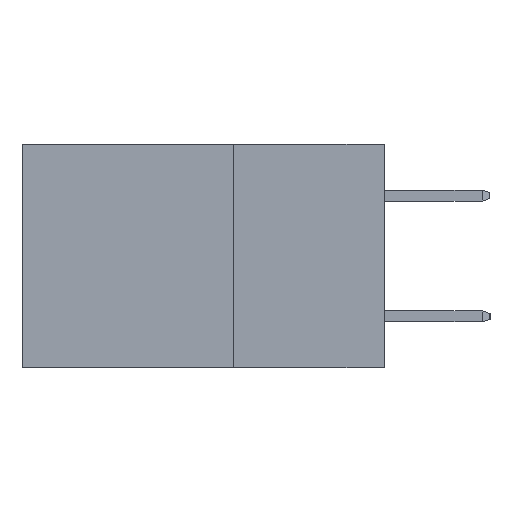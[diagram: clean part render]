
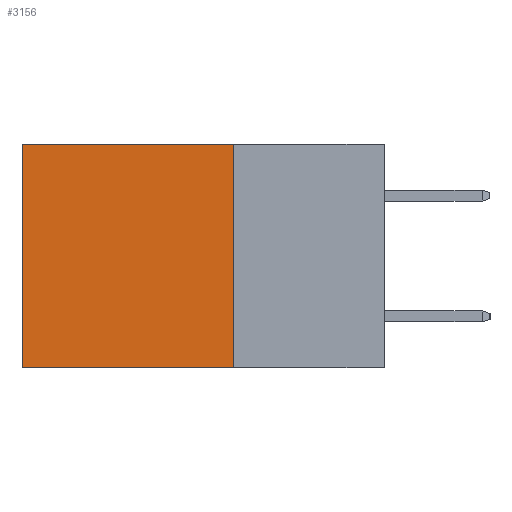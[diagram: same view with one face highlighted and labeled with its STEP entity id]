
A CAD part, left-side view. The second image highlights one B-rep face of the part: STEP entity #3156.
In plain terms, the highlighted planar face has unit normal (-1, 0, 0).
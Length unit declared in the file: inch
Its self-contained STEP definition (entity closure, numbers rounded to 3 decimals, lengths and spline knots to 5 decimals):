
#375 = ORIENTED_EDGE ( 'NONE', *, *, #1338, .T. ) ;
#456 = FACE_OUTER_BOUND ( 'NONE', #4893, .T. ) ;
#567 = DIRECTION ( 'NONE',  ( 0., 0., -1. ) ) ;
#1302 = DIRECTION ( 'NONE',  ( 1., 0., 0. ) ) ;
#1338 = EDGE_CURVE ( 'NONE', #3734, #2623, #2276, .T. ) ;
#1370 = CARTESIAN_POINT ( 'NONE',  ( 0.2615, 0.25, -0.37 ) ) ;
#1402 = VERTEX_POINT ( 'NONE', #6561 ) ;
#1409 = CARTESIAN_POINT ( 'NONE',  ( 0.2615, 0.25, 0. ) ) ;
#1435 = LINE ( 'NONE', #5054, #8711 ) ;
#1612 = EDGE_CURVE ( 'NONE', #2623, #4270, #5603, .T. ) ;
#1864 = DIRECTION ( 'NONE',  ( 0., 1., 0. ) ) ;
#2276 = LINE ( 'NONE', #5927, #5505 ) ;
#2623 = VERTEX_POINT ( 'NONE', #6834 ) ;
#3156 = ADVANCED_FACE ( 'NONE', ( #456 ), #7537, .F. ) ;
#3718 = VECTOR ( 'NONE', #5044, 39.37008 ) ;
#3734 = VERTEX_POINT ( 'NONE', #1409 ) ;
#4270 = VERTEX_POINT ( 'NONE', #4678 ) ;
#4388 = ORIENTED_EDGE ( 'NONE', *, *, #7783, .F. ) ;
#4629 = EDGE_CURVE ( 'NONE', #1402, #4270, #5745, .T. ) ;
#4678 = CARTESIAN_POINT ( 'NONE',  ( 0.2615, 0.6, -0.37 ) ) ;
#4829 = CARTESIAN_POINT ( 'NONE',  ( 0.2615, 0.6, -0.37 ) ) ;
#4893 = EDGE_LOOP ( 'NONE', ( #9048, #6938, #4388, #375 ) ) ;
#5044 = DIRECTION ( 'NONE',  ( 0., 0., -1. ) ) ;
#5054 = CARTESIAN_POINT ( 'NONE',  ( 0.2615, 0.25, -0.37 ) ) ;
#5505 = VECTOR ( 'NONE', #1864, 39.37008 ) ;
#5603 = LINE ( 'NONE', #4829, #3718 ) ;
#5745 = LINE ( 'NONE', #8118, #8995 ) ;
#5927 = CARTESIAN_POINT ( 'NONE',  ( 0.2615, 0.25, 0. ) ) ;
#6561 = CARTESIAN_POINT ( 'NONE',  ( 0.2615, 0.25, -0.37 ) ) ;
#6834 = CARTESIAN_POINT ( 'NONE',  ( 0.2615, 0.6, 0. ) ) ;
#6938 = ORIENTED_EDGE ( 'NONE', *, *, #4629, .F. ) ;
#7511 = AXIS2_PLACEMENT_3D ( 'NONE', #1370, #1302, #567 ) ;
#7537 = PLANE ( 'NONE',  #7511 ) ;
#7626 = DIRECTION ( 'NONE',  ( 0., 1., 0. ) ) ;
#7783 = EDGE_CURVE ( 'NONE', #3734, #1402, #1435, .T. ) ;
#8118 = CARTESIAN_POINT ( 'NONE',  ( 0.2615, 0.25, -0.37 ) ) ;
#8711 = VECTOR ( 'NONE', #8998, 39.37008 ) ;
#8995 = VECTOR ( 'NONE', #7626, 39.37008 ) ;
#8998 = DIRECTION ( 'NONE',  ( 0., 0., -1. ) ) ;
#9048 = ORIENTED_EDGE ( 'NONE', *, *, #1612, .T. ) ;
